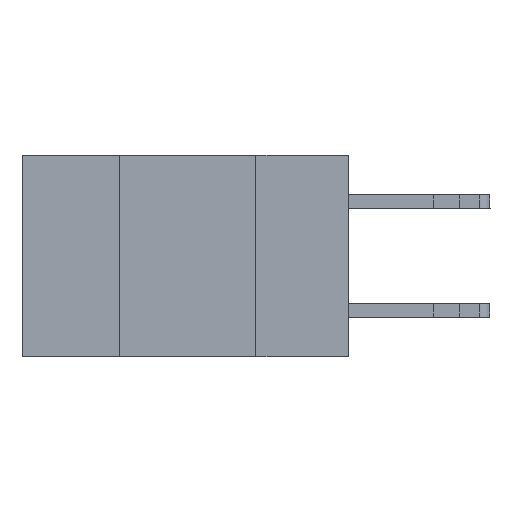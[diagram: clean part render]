
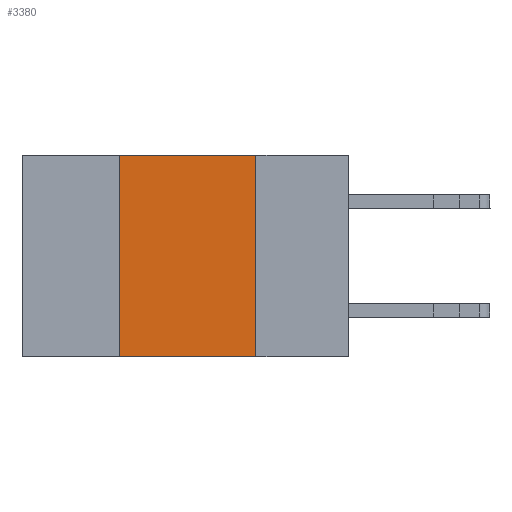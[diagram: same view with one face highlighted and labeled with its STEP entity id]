
A CAD part, left-side view. The second image highlights one B-rep face of the part: STEP entity #3380.
In plain terms, the highlighted planar face has unit normal (-1, 0, 0).
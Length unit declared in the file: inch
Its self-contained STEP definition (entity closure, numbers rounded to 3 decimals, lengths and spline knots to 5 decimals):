
#876 = ORIENTED_EDGE ( 'NONE', *, *, #4702, .T. ) ;
#908 = LINE ( 'NONE', #4346, #10466 ) ;
#949 = VERTEX_POINT ( 'NONE', #9259 ) ;
#1205 = LINE ( 'NONE', #4658, #11226 ) ;
#1701 = LINE ( 'NONE', #5104, #5869 ) ;
#1709 = FACE_OUTER_BOUND ( 'NONE', #4511, .T. ) ;
#3338 = DIRECTION ( 'NONE',  ( 0., -1., 0. ) ) ;
#3380 = ADVANCED_FACE ( 'NONE', ( #1709 ), #12723, .F. ) ;
#3571 = VECTOR ( 'NONE', #3338, 39.37008 ) ;
#3696 = VERTEX_POINT ( 'NONE', #6281 ) ;
#3760 = EDGE_CURVE ( 'NONE', #7259, #8648, #908, .T. ) ;
#3995 = CARTESIAN_POINT ( 'NONE',  ( 0., 0.6, 0. ) ) ;
#4133 = DIRECTION ( 'NONE',  ( 0., -1., 0. ) ) ;
#4346 = CARTESIAN_POINT ( 'NONE',  ( 0., 0.17, -0.37 ) ) ;
#4511 = EDGE_LOOP ( 'NONE', ( #10380, #12545, #8823, #876 ) ) ;
#4658 = CARTESIAN_POINT ( 'NONE',  ( 0., 0.42, -0.37 ) ) ;
#4702 = EDGE_CURVE ( 'NONE', #949, #8648, #1701, .T. ) ;
#5104 = CARTESIAN_POINT ( 'NONE',  ( 0., 0.6, -0.37 ) ) ;
#5869 = VECTOR ( 'NONE', #4133, 39.37008 ) ;
#6129 = EDGE_CURVE ( 'NONE', #949, #3696, #1205, .T. ) ;
#6281 = CARTESIAN_POINT ( 'NONE',  ( 0., 0.42, 0. ) ) ;
#7259 = VERTEX_POINT ( 'NONE', #11164 ) ;
#8648 = VERTEX_POINT ( 'NONE', #13949 ) ;
#8823 = ORIENTED_EDGE ( 'NONE', *, *, #6129, .F. ) ;
#9065 = DIRECTION ( 'NONE',  ( 0., 0., 1. ) ) ;
#9259 = CARTESIAN_POINT ( 'NONE',  ( 0., 0.42, -0.37 ) ) ;
#9800 = DIRECTION ( 'NONE',  ( 0., 0., -1. ) ) ;
#10250 = EDGE_CURVE ( 'NONE', #3696, #7259, #13922, .T. ) ;
#10380 = ORIENTED_EDGE ( 'NONE', *, *, #3760, .F. ) ;
#10466 = VECTOR ( 'NONE', #9800, 39.37008 ) ;
#10832 = DIRECTION ( 'NONE',  ( 1., 0., 0. ) ) ;
#11164 = CARTESIAN_POINT ( 'NONE',  ( 0., 0.17, 0. ) ) ;
#11226 = VECTOR ( 'NONE', #9065, 39.37008 ) ;
#11887 = AXIS2_PLACEMENT_3D ( 'NONE', #3995, #10832, #12951 ) ;
#12545 = ORIENTED_EDGE ( 'NONE', *, *, #10250, .F. ) ;
#12723 = PLANE ( 'NONE',  #11887 ) ;
#12951 = DIRECTION ( 'NONE',  ( 0., 0., -1. ) ) ;
#13922 = LINE ( 'NONE', #14073, #3571 ) ;
#13949 = CARTESIAN_POINT ( 'NONE',  ( 0., 0.17, -0.37 ) ) ;
#14073 = CARTESIAN_POINT ( 'NONE',  ( 0., 0.6, 0. ) ) ;
